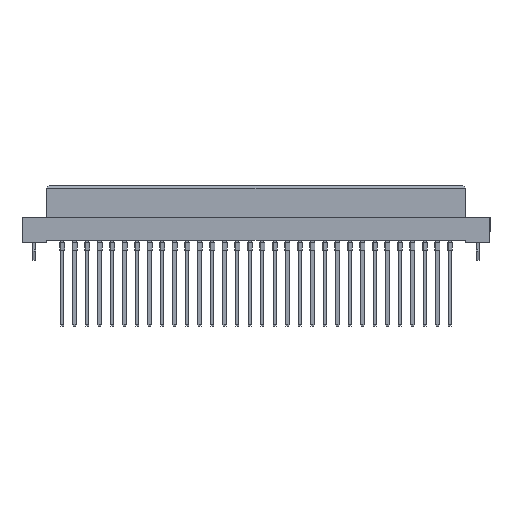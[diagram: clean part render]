
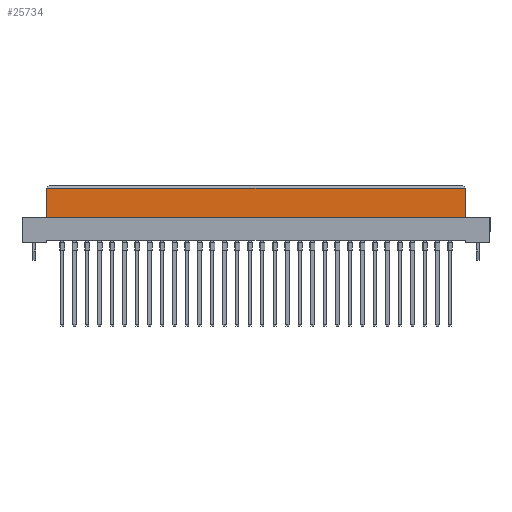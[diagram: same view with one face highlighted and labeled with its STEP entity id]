
A CAD part, top view. The second image highlights one B-rep face of the part: STEP entity #25734.
In plain terms, the highlighted planar face has unit normal (0, 0, 1).
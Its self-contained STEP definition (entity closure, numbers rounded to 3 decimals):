
#309 = DIRECTION ( 'NONE',  ( -1., 0., 0. ) ) ;
#1390 = DIRECTION ( 'NONE',  ( 0., 1., 0. ) ) ;
#1660 = EDGE_CURVE ( 'NONE', #26914, #33187, #14877, .T. ) ;
#2444 = CARTESIAN_POINT ( 'NONE',  ( -42.5, -6.4, 4.25 ) ) ;
#2708 = CARTESIAN_POINT ( 'NONE',  ( -42.5, -0.5, 4.25 ) ) ;
#2940 = VERTEX_POINT ( 'NONE', #39128 ) ;
#5602 = DIRECTION ( 'NONE',  ( 1., 0., 0. ) ) ;
#8372 = ORIENTED_EDGE ( 'NONE', *, *, #16307, .T. ) ;
#10447 = CARTESIAN_POINT ( 'NONE',  ( 42.5, -6.4, 4.25 ) ) ;
#10847 = FACE_OUTER_BOUND ( 'NONE', #17162, .T. ) ;
#14769 = LINE ( 'NONE', #26985, #24865 ) ;
#14877 = LINE ( 'NONE', #2444, #30951 ) ;
#14953 = VECTOR ( 'NONE', #1390, 1000. ) ;
#16307 = EDGE_CURVE ( 'NONE', #29093, #2940, #37515, .T. ) ;
#17162 = EDGE_LOOP ( 'NONE', ( #8372, #35680, #26633, #30064 ) ) ;
#17601 = EDGE_CURVE ( 'NONE', #26914, #29093, #14769, .T. ) ;
#18812 = EDGE_CURVE ( 'NONE', #2940, #33187, #33197, .T. ) ;
#23234 = DIRECTION ( 'NONE',  ( 0., 0., 1. ) ) ;
#24313 = CARTESIAN_POINT ( 'NONE',  ( -42.5, -0.5, 4.25 ) ) ;
#24865 = VECTOR ( 'NONE', #36195, 1000. ) ;
#25734 = ADVANCED_FACE ( 'NONE', ( #10847 ), #34283, .T. ) ;
#26262 = CARTESIAN_POINT ( 'NONE',  ( 42.5, -6.4, 4.25 ) ) ;
#26633 = ORIENTED_EDGE ( 'NONE', *, *, #1660, .F. ) ;
#26914 = VERTEX_POINT ( 'NONE', #38295 ) ;
#26985 = CARTESIAN_POINT ( 'NONE',  ( 42.5, -6.4, 4.25 ) ) ;
#27101 = DIRECTION ( 'NONE',  ( 0., 1., 0. ) ) ;
#29093 = VERTEX_POINT ( 'NONE', #35389 ) ;
#30064 = ORIENTED_EDGE ( 'NONE', *, *, #17601, .T. ) ;
#30951 = VECTOR ( 'NONE', #27101, 1000. ) ;
#32481 = AXIS2_PLACEMENT_3D ( 'NONE', #26262, #23234, #5602 ) ;
#33187 = VERTEX_POINT ( 'NONE', #24313 ) ;
#33197 = LINE ( 'NONE', #2708, #37088 ) ;
#34283 = PLANE ( 'NONE',  #32481 ) ;
#35389 = CARTESIAN_POINT ( 'NONE',  ( 42.5, -6.4, 4.25 ) ) ;
#35680 = ORIENTED_EDGE ( 'NONE', *, *, #18812, .T. ) ;
#36195 = DIRECTION ( 'NONE',  ( 1., 0., 0. ) ) ;
#37088 = VECTOR ( 'NONE', #309, 1000. ) ;
#37515 = LINE ( 'NONE', #10447, #14953 ) ;
#38295 = CARTESIAN_POINT ( 'NONE',  ( -42.5, -6.4, 4.25 ) ) ;
#39128 = CARTESIAN_POINT ( 'NONE',  ( 42.5, -0.5, 4.25 ) ) ;
